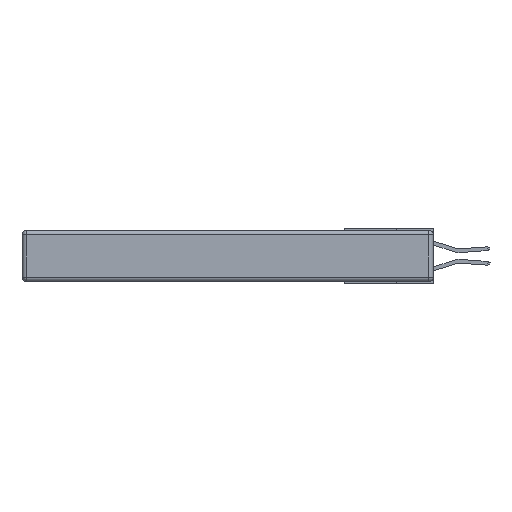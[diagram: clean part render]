
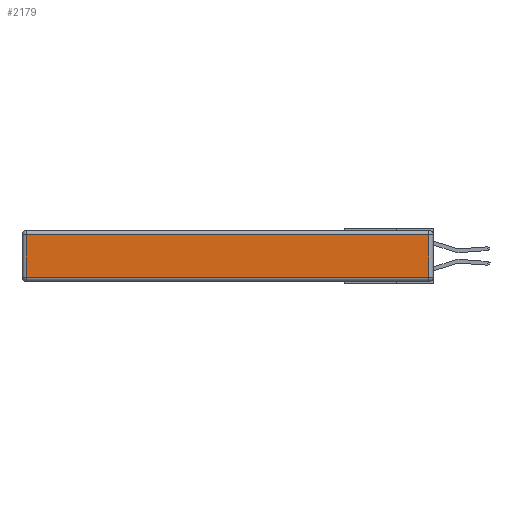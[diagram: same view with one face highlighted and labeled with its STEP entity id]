
A CAD part, left-side view. The second image highlights one B-rep face of the part: STEP entity #2179.
In plain terms, the highlighted planar face has unit normal (-1, 0, 0).
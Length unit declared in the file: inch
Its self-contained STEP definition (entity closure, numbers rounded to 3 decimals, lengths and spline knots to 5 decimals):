
#679 = VECTOR ( 'NONE', #10175, 39.37008 ) ;
#1350 = DIRECTION ( 'NONE',  ( 0., 0., 1. ) ) ;
#1702 = ORIENTED_EDGE ( 'NONE', *, *, #7819, .T. ) ;
#2138 = ORIENTED_EDGE ( 'NONE', *, *, #3738, .T. ) ;
#2179 = ADVANCED_FACE ( 'NONE', ( #7751 ), #7566, .T. ) ;
#2563 = VECTOR ( 'NONE', #7501, 39.37008 ) ;
#2826 = EDGE_CURVE ( 'NONE', #6677, #6337, #3933, .T. ) ;
#3110 = CARTESIAN_POINT ( 'NONE',  ( 0., 0.03, -0.343 ) ) ;
#3440 = ORIENTED_EDGE ( 'NONE', *, *, #2826, .T. ) ;
#3738 = EDGE_CURVE ( 'NONE', #8263, #12681, #7685, .T. ) ;
#3933 = LINE ( 'NONE', #7205, #11603 ) ;
#4833 = LINE ( 'NONE', #12730, #2563 ) ;
#5998 = CARTESIAN_POINT ( 'NONE',  ( 0., 2.75, -0.03 ) ) ;
#6157 = DIRECTION ( 'NONE',  ( 0., 0., 1. ) ) ;
#6337 = VERTEX_POINT ( 'NONE', #12691 ) ;
#6600 = DIRECTION ( 'NONE',  ( -1., 0., 0. ) ) ;
#6677 = VERTEX_POINT ( 'NONE', #11873 ) ;
#7205 = CARTESIAN_POINT ( 'NONE',  ( 0., 0., -0.313 ) ) ;
#7391 = EDGE_CURVE ( 'NONE', #12681, #6677, #4833, .T. ) ;
#7501 = DIRECTION ( 'NONE',  ( 0., 0., -1. ) ) ;
#7566 = PLANE ( 'NONE',  #10657 ) ;
#7685 = LINE ( 'NONE', #5998, #679 ) ;
#7751 = FACE_OUTER_BOUND ( 'NONE', #11640, .T. ) ;
#7819 = EDGE_CURVE ( 'NONE', #6337, #8263, #10665, .T. ) ;
#8263 = VERTEX_POINT ( 'NONE', #10992 ) ;
#9021 = ORIENTED_EDGE ( 'NONE', *, *, #7391, .T. ) ;
#9709 = VECTOR ( 'NONE', #6157, 39.37008 ) ;
#10175 = DIRECTION ( 'NONE',  ( 0., 1., 0. ) ) ;
#10375 = DIRECTION ( 'NONE',  ( 0., -1., 0. ) ) ;
#10657 = AXIS2_PLACEMENT_3D ( 'NONE', #10741, #6600, #1350 ) ;
#10665 = LINE ( 'NONE', #3110, #9709 ) ;
#10741 = CARTESIAN_POINT ( 'NONE',  ( 0., 0., -0.343 ) ) ;
#10992 = CARTESIAN_POINT ( 'NONE',  ( 0., 0.03, -0.03 ) ) ;
#11603 = VECTOR ( 'NONE', #10375, 39.37008 ) ;
#11635 = CARTESIAN_POINT ( 'NONE',  ( 0., 2.72, -0.03 ) ) ;
#11640 = EDGE_LOOP ( 'NONE', ( #3440, #1702, #2138, #9021 ) ) ;
#11873 = CARTESIAN_POINT ( 'NONE',  ( 0., 2.72, -0.313 ) ) ;
#12681 = VERTEX_POINT ( 'NONE', #11635 ) ;
#12691 = CARTESIAN_POINT ( 'NONE',  ( 0., 0.03, -0.313 ) ) ;
#12730 = CARTESIAN_POINT ( 'NONE',  ( 0., 2.72, -0.343 ) ) ;
